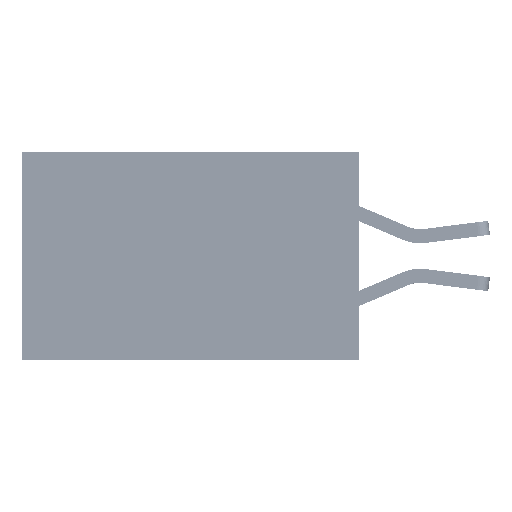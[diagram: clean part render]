
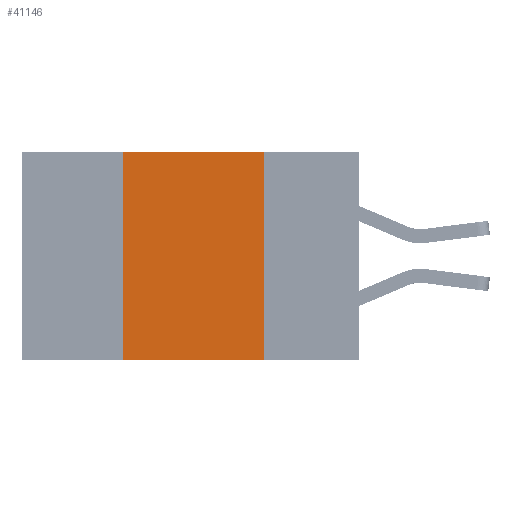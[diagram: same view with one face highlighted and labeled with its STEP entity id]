
A CAD part, left-side view. The second image highlights one B-rep face of the part: STEP entity #41146.
In plain terms, the highlighted planar face has unit normal (-1, 0, 0).
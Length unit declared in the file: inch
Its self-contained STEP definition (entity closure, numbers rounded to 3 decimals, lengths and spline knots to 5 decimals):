
#106 = EDGE_CURVE ( 'NONE', #39617, #12693, #553, .T. ) ;
#553 = LINE ( 'NONE', #24933, #37648 ) ;
#572 = ORIENTED_EDGE ( 'NONE', *, *, #106, .F. ) ;
#1416 = CARTESIAN_POINT ( 'NONE',  ( 0., 0.6, 0. ) ) ;
#3639 = EDGE_CURVE ( 'NONE', #23194, #39617, #25344, .T. ) ;
#4820 = ORIENTED_EDGE ( 'NONE', *, *, #29313, .T. ) ;
#7266 = CARTESIAN_POINT ( 'NONE',  ( 0., 0.17, 0. ) ) ;
#8344 = DIRECTION ( 'NONE',  ( 0., -1., 0. ) ) ;
#11883 = LINE ( 'NONE', #24072, #43030 ) ;
#12693 = VERTEX_POINT ( 'NONE', #32434 ) ;
#12922 = CARTESIAN_POINT ( 'NONE',  ( 0., 0.42, -0.37 ) ) ;
#14832 = VERTEX_POINT ( 'NONE', #12922 ) ;
#19562 = ORIENTED_EDGE ( 'NONE', *, *, #35584, .F. ) ;
#19583 = AXIS2_PLACEMENT_3D ( 'NONE', #40753, #33874, #23632 ) ;
#21679 = LINE ( 'NONE', #29673, #23826 ) ;
#23054 = DIRECTION ( 'NONE',  ( 0., -1., 0. ) ) ;
#23194 = VERTEX_POINT ( 'NONE', #40536 ) ;
#23348 = PLANE ( 'NONE',  #19583 ) ;
#23632 = DIRECTION ( 'NONE',  ( 0., 0., -1. ) ) ;
#23826 = VECTOR ( 'NONE', #23054, 39.37008 ) ;
#24072 = CARTESIAN_POINT ( 'NONE',  ( 0., 0.42, 0. ) ) ;
#24933 = CARTESIAN_POINT ( 'NONE',  ( 0., 0.17, 0. ) ) ;
#25344 = LINE ( 'NONE', #1416, #40916 ) ;
#28566 = DIRECTION ( 'NONE',  ( 0., 0., -1. ) ) ;
#29313 = EDGE_CURVE ( 'NONE', #14832, #12693, #21679, .T. ) ;
#29673 = CARTESIAN_POINT ( 'NONE',  ( 0., 0.6, -0.37 ) ) ;
#29993 = FACE_OUTER_BOUND ( 'NONE', #42094, .T. ) ;
#31001 = DIRECTION ( 'NONE',  ( 0., 0., 1. ) ) ;
#32434 = CARTESIAN_POINT ( 'NONE',  ( 0., 0.17, -0.37 ) ) ;
#33874 = DIRECTION ( 'NONE',  ( 1., 0., 0. ) ) ;
#35584 = EDGE_CURVE ( 'NONE', #14832, #23194, #11883, .T. ) ;
#37648 = VECTOR ( 'NONE', #28566, 39.37008 ) ;
#38732 = ORIENTED_EDGE ( 'NONE', *, *, #3639, .F. ) ;
#39617 = VERTEX_POINT ( 'NONE', #7266 ) ;
#40536 = CARTESIAN_POINT ( 'NONE',  ( 0., 0.42, 0. ) ) ;
#40753 = CARTESIAN_POINT ( 'NONE',  ( 0., 0.6, 0. ) ) ;
#40916 = VECTOR ( 'NONE', #8344, 39.37008 ) ;
#41146 = ADVANCED_FACE ( 'NONE', ( #29993 ), #23348, .F. ) ;
#42094 = EDGE_LOOP ( 'NONE', ( #572, #38732, #19562, #4820 ) ) ;
#43030 = VECTOR ( 'NONE', #31001, 39.37008 ) ;
